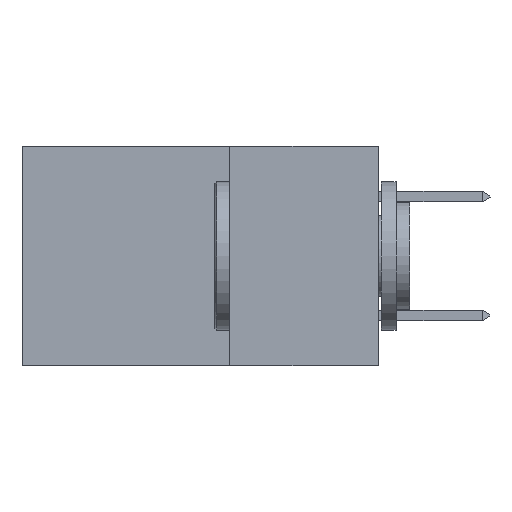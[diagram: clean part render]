
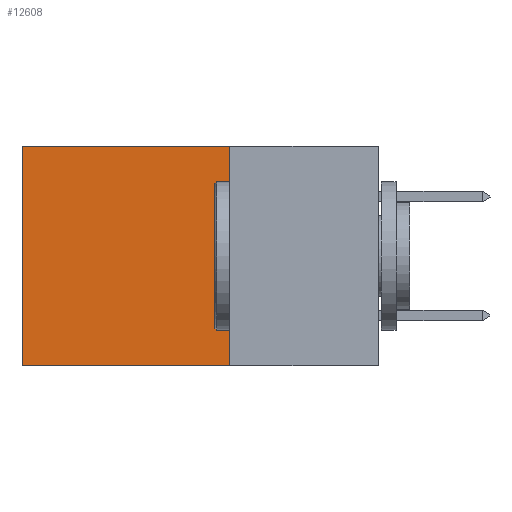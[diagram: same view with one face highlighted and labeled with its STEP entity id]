
A CAD part, left-side view. The second image highlights one B-rep face of the part: STEP entity #12608.
In plain terms, the highlighted planar face has unit normal (-1, 0, 0).
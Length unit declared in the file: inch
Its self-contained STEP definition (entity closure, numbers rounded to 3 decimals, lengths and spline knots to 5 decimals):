
#1544 = CARTESIAN_POINT ( 'NONE',  ( 0.298, 0.25, -0.37 ) ) ;
#3140 = CARTESIAN_POINT ( 'NONE',  ( 0.298, 0.25, 0. ) ) ;
#3763 = DIRECTION ( 'NONE',  ( 1., 0., 0. ) ) ;
#4780 = VERTEX_POINT ( 'NONE', #23971 ) ;
#5391 = EDGE_CURVE ( 'NONE', #7791, #18833, #11900, .T. ) ;
#5611 = VECTOR ( 'NONE', #11158, 39.37008 ) ;
#7475 = AXIS2_PLACEMENT_3D ( 'NONE', #22764, #3763, #20770 ) ;
#7529 = VERTEX_POINT ( 'NONE', #25858 ) ;
#7573 = EDGE_CURVE ( 'NONE', #7529, #4780, #24945, .T. ) ;
#7621 = DIRECTION ( 'NONE',  ( 0., 1., 0. ) ) ;
#7791 = VERTEX_POINT ( 'NONE', #20523 ) ;
#8084 = CARTESIAN_POINT ( 'NONE',  ( 0.298, 0.6, -0.37 ) ) ;
#10015 = PLANE ( 'NONE',  #7475 ) ;
#10973 = CARTESIAN_POINT ( 'NONE',  ( 0.298, 0.6, 0. ) ) ;
#11158 = DIRECTION ( 'NONE',  ( 0., 0., -1. ) ) ;
#11900 = LINE ( 'NONE', #1544, #25845 ) ;
#12098 = LINE ( 'NONE', #10973, #5611 ) ;
#12608 = ADVANCED_FACE ( 'NONE', ( #17677 ), #10015, .F. ) ;
#13137 = EDGE_CURVE ( 'NONE', #4780, #18833, #12098, .T. ) ;
#14472 = VECTOR ( 'NONE', #25044, 39.37008 ) ;
#17677 = FACE_OUTER_BOUND ( 'NONE', #21391, .T. ) ;
#18014 = ORIENTED_EDGE ( 'NONE', *, *, #13137, .T. ) ;
#18833 = VERTEX_POINT ( 'NONE', #8084 ) ;
#20013 = LINE ( 'NONE', #22976, #14472 ) ;
#20523 = CARTESIAN_POINT ( 'NONE',  ( 0.298, 0.25, -0.37 ) ) ;
#20770 = DIRECTION ( 'NONE',  ( 0., 0., -1. ) ) ;
#20873 = ORIENTED_EDGE ( 'NONE', *, *, #25261, .F. ) ;
#21391 = EDGE_LOOP ( 'NONE', ( #18014, #26860, #20873, #23955 ) ) ;
#22764 = CARTESIAN_POINT ( 'NONE',  ( 0.298, 0.25, 0. ) ) ;
#22976 = CARTESIAN_POINT ( 'NONE',  ( 0.298, 0.25, 0. ) ) ;
#23955 = ORIENTED_EDGE ( 'NONE', *, *, #7573, .T. ) ;
#23971 = CARTESIAN_POINT ( 'NONE',  ( 0.298, 0.6, 0. ) ) ;
#24637 = VECTOR ( 'NONE', #7621, 39.37008 ) ;
#24945 = LINE ( 'NONE', #3140, #24637 ) ;
#25044 = DIRECTION ( 'NONE',  ( 0., 0., -1. ) ) ;
#25261 = EDGE_CURVE ( 'NONE', #7529, #7791, #20013, .T. ) ;
#25845 = VECTOR ( 'NONE', #26258, 39.37008 ) ;
#25858 = CARTESIAN_POINT ( 'NONE',  ( 0.298, 0.25, 0. ) ) ;
#26258 = DIRECTION ( 'NONE',  ( 0., 1., 0. ) ) ;
#26860 = ORIENTED_EDGE ( 'NONE', *, *, #5391, .F. ) ;
